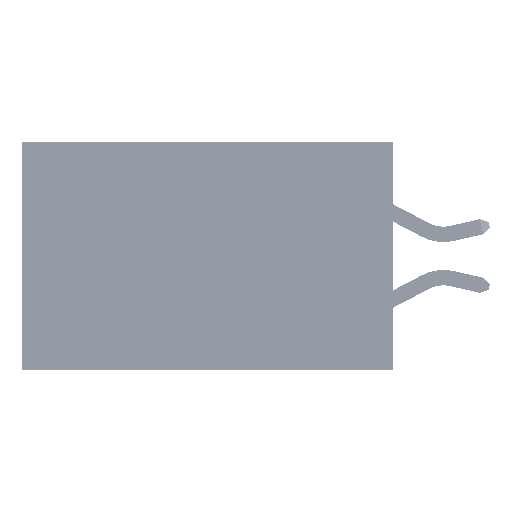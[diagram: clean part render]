
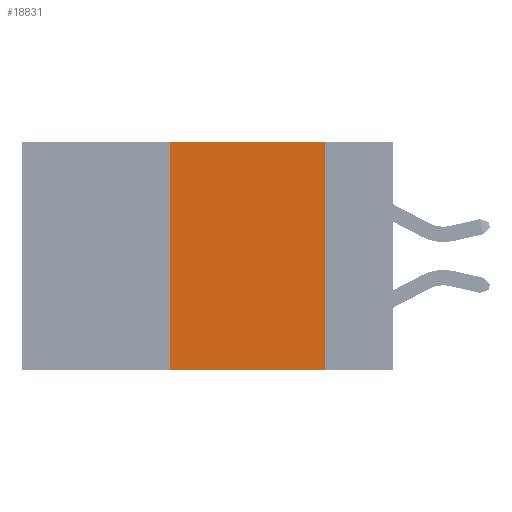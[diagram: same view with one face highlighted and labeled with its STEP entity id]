
A CAD part, left-side view. The second image highlights one B-rep face of the part: STEP entity #18831.
In plain terms, the highlighted planar face has unit normal (-1, 0, 0).
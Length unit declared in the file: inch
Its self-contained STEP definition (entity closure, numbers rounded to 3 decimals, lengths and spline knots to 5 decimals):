
#48 = CARTESIAN_POINT ( 'NONE',  ( 0., 0.6, 0. ) ) ;
#1351 = DIRECTION ( 'NONE',  ( 0., -1., 0. ) ) ;
#1781 = LINE ( 'NONE', #26533, #50521 ) ;
#1963 = LINE ( 'NONE', #13693, #3086 ) ;
#2455 = VERTEX_POINT ( 'NONE', #19742 ) ;
#3086 = VECTOR ( 'NONE', #42483, 39.37008 ) ;
#3883 = CARTESIAN_POINT ( 'NONE',  ( 0., 0.36, 0. ) ) ;
#4030 = ORIENTED_EDGE ( 'NONE', *, *, #42093, .F. ) ;
#6255 = ORIENTED_EDGE ( 'NONE', *, *, #36896, .F. ) ;
#9299 = VERTEX_POINT ( 'NONE', #10808 ) ;
#10808 = CARTESIAN_POINT ( 'NONE',  ( 0., 0.11, -0.37 ) ) ;
#13693 = CARTESIAN_POINT ( 'NONE',  ( 0., 0.6, 0. ) ) ;
#14326 = EDGE_LOOP ( 'NONE', ( #36230, #6255, #4030, #20342 ) ) ;
#17566 = VERTEX_POINT ( 'NONE', #18718 ) ;
#18718 = CARTESIAN_POINT ( 'NONE',  ( 0., 0.36, -0.37 ) ) ;
#18831 = ADVANCED_FACE ( 'NONE', ( #29299 ), #20531, .F. ) ;
#19742 = CARTESIAN_POINT ( 'NONE',  ( 0., 0.36, 0. ) ) ;
#20342 = ORIENTED_EDGE ( 'NONE', *, *, #49954, .T. ) ;
#20531 = PLANE ( 'NONE',  #32168 ) ;
#20712 = CARTESIAN_POINT ( 'NONE',  ( 0., 0.11, 0. ) ) ;
#24373 = DIRECTION ( 'NONE',  ( 0., 0., 1. ) ) ;
#26533 = CARTESIAN_POINT ( 'NONE',  ( 0., 0.11, 0. ) ) ;
#26750 = VECTOR ( 'NONE', #1351, 39.37008 ) ;
#29299 = FACE_OUTER_BOUND ( 'NONE', #14326, .T. ) ;
#29740 = DIRECTION ( 'NONE',  ( 0., 0., -1. ) ) ;
#31402 = VERTEX_POINT ( 'NONE', #20712 ) ;
#31569 = LINE ( 'NONE', #3883, #49449 ) ;
#31618 = EDGE_CURVE ( 'NONE', #31402, #9299, #1781, .T. ) ;
#32168 = AXIS2_PLACEMENT_3D ( 'NONE', #48, #41603, #32780 ) ;
#32780 = DIRECTION ( 'NONE',  ( 0., 0., -1. ) ) ;
#36230 = ORIENTED_EDGE ( 'NONE', *, *, #31618, .F. ) ;
#36896 = EDGE_CURVE ( 'NONE', #2455, #31402, #1963, .T. ) ;
#41603 = DIRECTION ( 'NONE',  ( 1., 0., 0. ) ) ;
#41872 = CARTESIAN_POINT ( 'NONE',  ( 0., 0.6, -0.37 ) ) ;
#42093 = EDGE_CURVE ( 'NONE', #17566, #2455, #31569, .T. ) ;
#42144 = LINE ( 'NONE', #41872, #26750 ) ;
#42483 = DIRECTION ( 'NONE',  ( 0., -1., 0. ) ) ;
#49449 = VECTOR ( 'NONE', #24373, 39.37008 ) ;
#49954 = EDGE_CURVE ( 'NONE', #17566, #9299, #42144, .T. ) ;
#50521 = VECTOR ( 'NONE', #29740, 39.37008 ) ;
